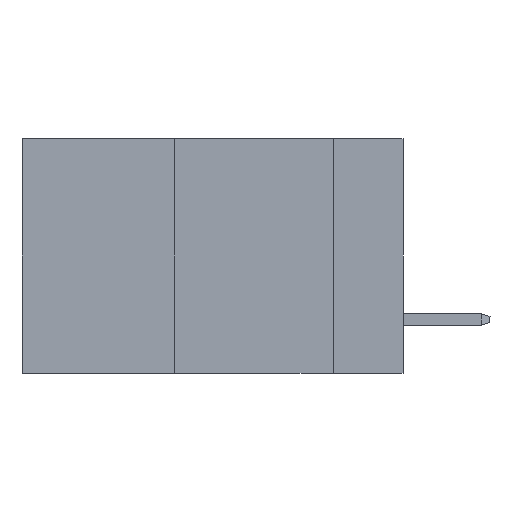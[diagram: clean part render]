
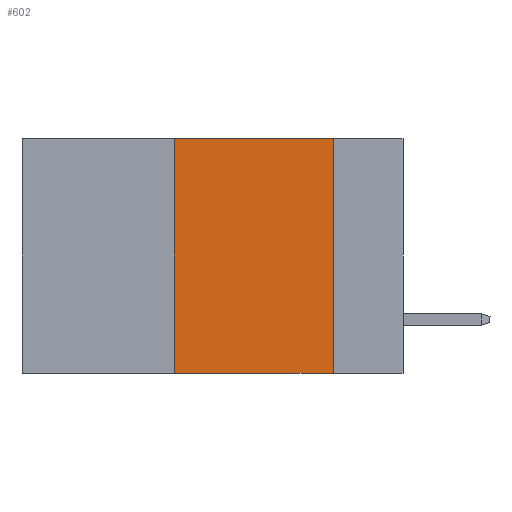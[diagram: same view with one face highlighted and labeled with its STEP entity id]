
A CAD part, left-side view. The second image highlights one B-rep face of the part: STEP entity #602.
In plain terms, the highlighted planar face has unit normal (-1, 0, 0).
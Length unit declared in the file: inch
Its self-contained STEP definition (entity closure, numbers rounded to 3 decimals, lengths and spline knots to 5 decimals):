
#304 = VECTOR ( 'NONE', #9230, 39.37008 ) ;
#395 = CARTESIAN_POINT ( 'NONE',  ( 0., 0.6, -0.37 ) ) ;
#478 = VERTEX_POINT ( 'NONE', #9459 ) ;
#602 = ADVANCED_FACE ( 'NONE', ( #1616 ), #752, .F. ) ;
#752 = PLANE ( 'NONE',  #1325 ) ;
#872 = ORIENTED_EDGE ( 'NONE', *, *, #6764, .F. ) ;
#1037 = ORIENTED_EDGE ( 'NONE', *, *, #9652, .F. ) ;
#1161 = EDGE_LOOP ( 'NONE', ( #1037, #872, #8386, #7501 ) ) ;
#1266 = VECTOR ( 'NONE', #4459, 39.37008 ) ;
#1325 = AXIS2_PLACEMENT_3D ( 'NONE', #4026, #3099, #3929 ) ;
#1616 = FACE_OUTER_BOUND ( 'NONE', #1161, .T. ) ;
#3099 = DIRECTION ( 'NONE',  ( 1., 0., 0. ) ) ;
#3364 = VECTOR ( 'NONE', #9767, 39.37008 ) ;
#3818 = CARTESIAN_POINT ( 'NONE',  ( 0., 0.36, 0. ) ) ;
#3929 = DIRECTION ( 'NONE',  ( 0., 0., -1. ) ) ;
#4026 = CARTESIAN_POINT ( 'NONE',  ( 0., 0.6, 0. ) ) ;
#4335 = EDGE_CURVE ( 'NONE', #478, #9589, #8845, .T. ) ;
#4410 = LINE ( 'NONE', #4659, #1266 ) ;
#4459 = DIRECTION ( 'NONE',  ( 0., 0., 1. ) ) ;
#4659 = CARTESIAN_POINT ( 'NONE',  ( 0., 0.36, 0. ) ) ;
#5454 = CARTESIAN_POINT ( 'NONE',  ( 0., 0.11, -0.37 ) ) ;
#6036 = VERTEX_POINT ( 'NONE', #6243 ) ;
#6243 = CARTESIAN_POINT ( 'NONE',  ( 0., 0.11, 0. ) ) ;
#6764 = EDGE_CURVE ( 'NONE', #9610, #6036, #7795, .T. ) ;
#6837 = DIRECTION ( 'NONE',  ( 0., -1., 0. ) ) ;
#7040 = CARTESIAN_POINT ( 'NONE',  ( 0., 0.6, 0. ) ) ;
#7066 = CARTESIAN_POINT ( 'NONE',  ( 0., 0.11, 0. ) ) ;
#7313 = VECTOR ( 'NONE', #6837, 39.37008 ) ;
#7501 = ORIENTED_EDGE ( 'NONE', *, *, #4335, .T. ) ;
#7795 = LINE ( 'NONE', #7040, #7313 ) ;
#8386 = ORIENTED_EDGE ( 'NONE', *, *, #8833, .F. ) ;
#8833 = EDGE_CURVE ( 'NONE', #478, #9610, #4410, .T. ) ;
#8845 = LINE ( 'NONE', #395, #3364 ) ;
#9230 = DIRECTION ( 'NONE',  ( 0., 0., -1. ) ) ;
#9459 = CARTESIAN_POINT ( 'NONE',  ( 0., 0.36, -0.37 ) ) ;
#9589 = VERTEX_POINT ( 'NONE', #5454 ) ;
#9610 = VERTEX_POINT ( 'NONE', #3818 ) ;
#9652 = EDGE_CURVE ( 'NONE', #6036, #9589, #10023, .T. ) ;
#9767 = DIRECTION ( 'NONE',  ( 0., -1., 0. ) ) ;
#10023 = LINE ( 'NONE', #7066, #304 ) ;
